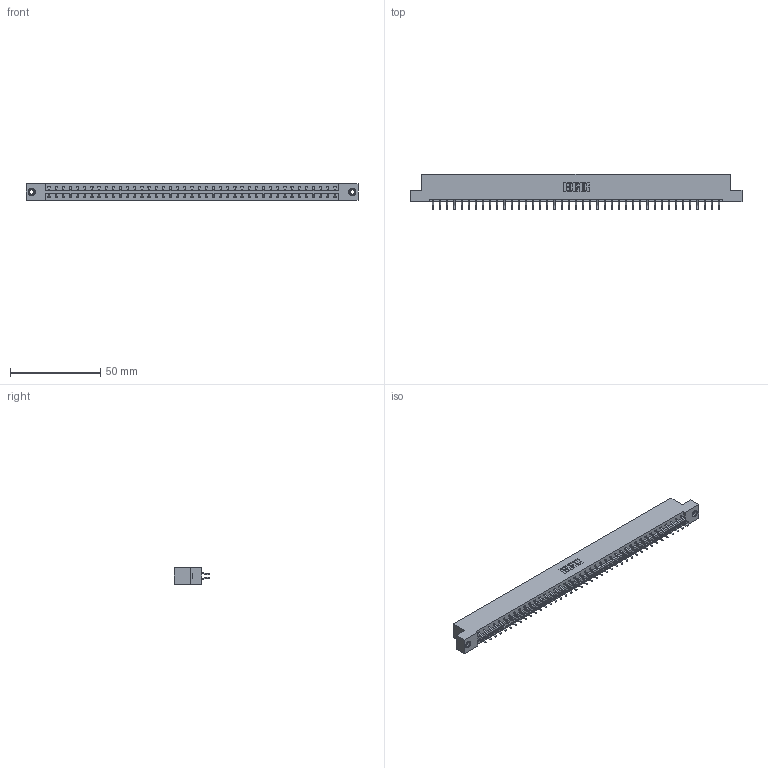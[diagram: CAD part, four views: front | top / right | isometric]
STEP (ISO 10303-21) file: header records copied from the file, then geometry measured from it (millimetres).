
FILE_DESCRIPTION (( 'STEP AP203' ), '1' );
FILE_NAME ('333-082-556-207.STEP', '2018-08-05T03:31:06', ( '' ), ( '' ), 'SwSTEP 2.0', 'SolidWorks 2016', '' );
FILE_SCHEMA (( 'CONFIG_CONTROL_DESIGN' ));
Length unit declared in the file: inch
Products named in the file (4): 345-292-001_556 Tail; 345-250-001_345-250-005-103; 333-082-556-207; 333 Part_Flush - .156 Dia - TI
Assembly tree (85 placements, depth 2):
  333-082-556-207
    333 Part_Flush - .156 Dia - TI
    345-292-001_556 Tail  x82
    345-250-001_345-250-005-103  x2
Bounding box: 184 x 19.57 x 9.4 mm (x, y, z)
Volume: 18759 mm3; surface area: 22120.3 mm2
Topology: 85 solids, 85 shells, 4930 faces, 14633 edges, 9638 vertices
Faces by surface type: plane 3382, cylinder 1532, cone 12, torus 4
Entity records: 27912 total; most frequent: CARTESIAN_POINT 4625, ORIENTED_EDGE 4542, DIRECTION 3973, EDGE_CURVE 2271, VECTOR 2115, LINE 2115, VERTEX_POINT 1508, AXIS2_PLACEMENT_3D 929
